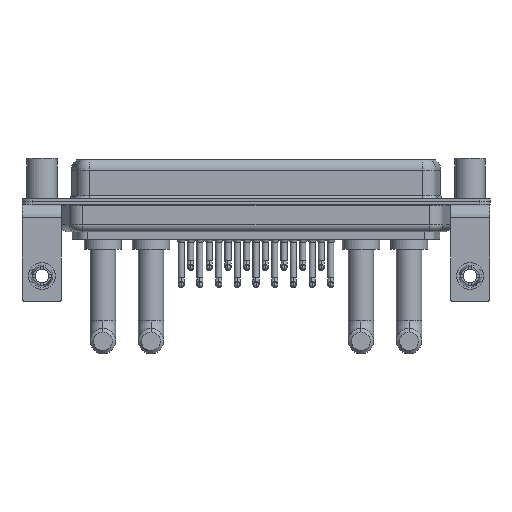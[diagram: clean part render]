
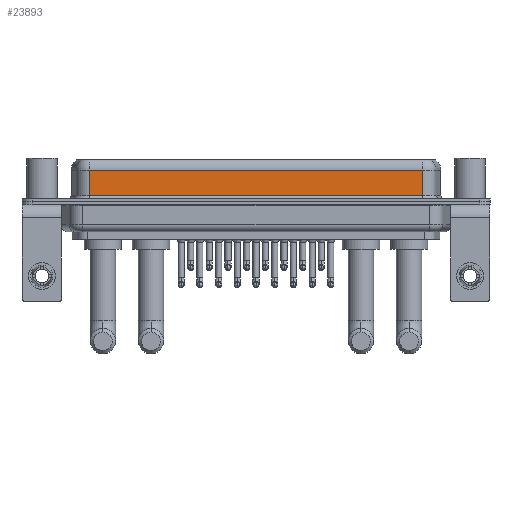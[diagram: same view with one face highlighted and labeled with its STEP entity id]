
A CAD part, front view. The second image highlights one B-rep face of the part: STEP entity #23893.
In plain terms, the highlighted planar face has unit normal (0, -1, 0).
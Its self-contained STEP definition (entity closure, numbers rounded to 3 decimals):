
#969 = EDGE_CURVE ( 'NONE', #6622, #18781, #2003, .T. ) ;
#2003 = LINE ( 'NONE', #19610, #16143 ) ;
#3381 = VERTEX_POINT ( 'NONE', #12835 ) ;
#3890 = CARTESIAN_POINT ( 'NONE',  ( 56.462, -3.95, 6.4 ) ) ;
#4016 = EDGE_CURVE ( 'NONE', #6622, #3381, #17211, .T. ) ;
#4897 = LINE ( 'NONE', #16675, #9764 ) ;
#6622 = VERTEX_POINT ( 'NONE', #18535 ) ;
#7086 = CARTESIAN_POINT ( 'NONE',  ( 7.038, -3.95, 0.9 ) ) ;
#9764 = VECTOR ( 'NONE', #24550, 1000. ) ;
#9945 = EDGE_LOOP ( 'NONE', ( #22702, #24914, #16943, #14751 ) ) ;
#10885 = LINE ( 'NONE', #12836, #18487 ) ;
#11967 = AXIS2_PLACEMENT_3D ( 'NONE', #3890, #23150, #13190 ) ;
#12835 = CARTESIAN_POINT ( 'NONE',  ( 56.462, -3.95, 0.9 ) ) ;
#12836 = CARTESIAN_POINT ( 'NONE',  ( 56.462, -3.95, 0.9 ) ) ;
#13190 = DIRECTION ( 'NONE',  ( 0., 0., 1. ) ) ;
#13523 = EDGE_CURVE ( 'NONE', #18781, #22390, #4897, .T. ) ;
#14751 = ORIENTED_EDGE ( 'NONE', *, *, #21886, .T. ) ;
#15412 = CARTESIAN_POINT ( 'NONE',  ( 7.038, -3.95, 4.65 ) ) ;
#15516 = FACE_OUTER_BOUND ( 'NONE', #9945, .T. ) ;
#16143 = VECTOR ( 'NONE', #17662, 1000. ) ;
#16675 = CARTESIAN_POINT ( 'NONE',  ( 7.038, -3.95, 6.4 ) ) ;
#16941 = DIRECTION ( 'NONE',  ( 0., 0., -1. ) ) ;
#16943 = ORIENTED_EDGE ( 'NONE', *, *, #13523, .T. ) ;
#17211 = LINE ( 'NONE', #23020, #20159 ) ;
#17662 = DIRECTION ( 'NONE',  ( -1., 0., 0. ) ) ;
#18487 = VECTOR ( 'NONE', #20481, 1000. ) ;
#18535 = CARTESIAN_POINT ( 'NONE',  ( 56.462, -3.95, 4.65 ) ) ;
#18781 = VERTEX_POINT ( 'NONE', #15412 ) ;
#19610 = CARTESIAN_POINT ( 'NONE',  ( 56.462, -3.95, 4.65 ) ) ;
#20159 = VECTOR ( 'NONE', #16941, 1000. ) ;
#20481 = DIRECTION ( 'NONE',  ( 1., 0., 0. ) ) ;
#21359 = PLANE ( 'NONE',  #11967 ) ;
#21886 = EDGE_CURVE ( 'NONE', #22390, #3381, #10885, .T. ) ;
#22390 = VERTEX_POINT ( 'NONE', #7086 ) ;
#22702 = ORIENTED_EDGE ( 'NONE', *, *, #4016, .F. ) ;
#23020 = CARTESIAN_POINT ( 'NONE',  ( 56.462, -3.95, 6.4 ) ) ;
#23150 = DIRECTION ( 'NONE',  ( 0., 1., 0. ) ) ;
#23893 = ADVANCED_FACE ( 'NONE', ( #15516 ), #21359, .F. ) ;
#24550 = DIRECTION ( 'NONE',  ( 0., 0., -1. ) ) ;
#24914 = ORIENTED_EDGE ( 'NONE', *, *, #969, .T. ) ;
